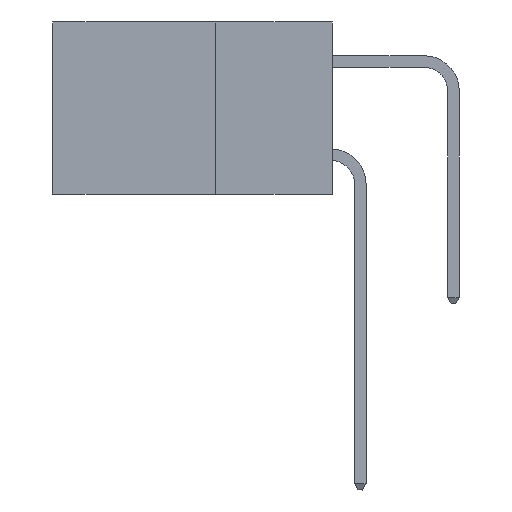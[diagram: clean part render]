
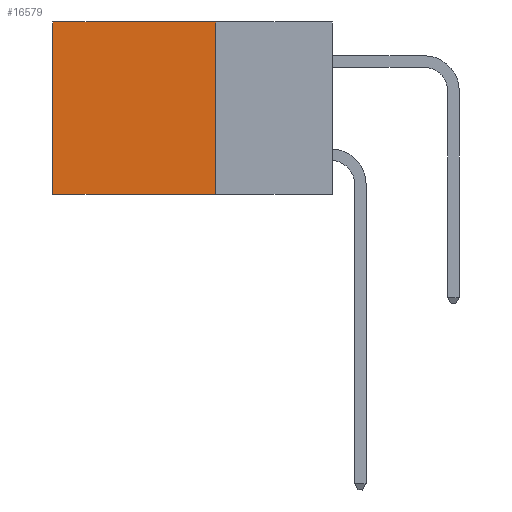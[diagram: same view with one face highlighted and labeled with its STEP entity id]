
A CAD part, left-side view. The second image highlights one B-rep face of the part: STEP entity #16579.
In plain terms, the highlighted planar face has unit normal (-1, 0, 0).
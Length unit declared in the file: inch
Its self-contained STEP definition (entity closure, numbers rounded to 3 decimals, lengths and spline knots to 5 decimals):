
#333 = CARTESIAN_POINT ( 'NONE',  ( 0.298, 0.25, 0. ) ) ;
#1179 = CARTESIAN_POINT ( 'NONE',  ( 0.298, 0.6, 0. ) ) ;
#1319 = VERTEX_POINT ( 'NONE', #1179 ) ;
#2018 = CARTESIAN_POINT ( 'NONE',  ( 0.298, 0.25, 0. ) ) ;
#2697 = VERTEX_POINT ( 'NONE', #4844 ) ;
#3037 = EDGE_LOOP ( 'NONE', ( #7070, #7316, #4612, #20606 ) ) ;
#3149 = LINE ( 'NONE', #3221, #21621 ) ;
#3221 = CARTESIAN_POINT ( 'NONE',  ( 0.298, 0.6, 0. ) ) ;
#4056 = EDGE_CURVE ( 'NONE', #14221, #2697, #16907, .T. ) ;
#4612 = ORIENTED_EDGE ( 'NONE', *, *, #23032, .F. ) ;
#4844 = CARTESIAN_POINT ( 'NONE',  ( 0.298, 0.6, -0.37 ) ) ;
#5186 = EDGE_CURVE ( 'NONE', #1319, #2697, #3149, .T. ) ;
#5882 = FACE_OUTER_BOUND ( 'NONE', #3037, .T. ) ;
#6401 = LINE ( 'NONE', #333, #12344 ) ;
#6707 = EDGE_CURVE ( 'NONE', #17365, #1319, #6401, .T. ) ;
#7070 = ORIENTED_EDGE ( 'NONE', *, *, #5186, .T. ) ;
#7260 = CARTESIAN_POINT ( 'NONE',  ( 0.298, 0.25, 0. ) ) ;
#7316 = ORIENTED_EDGE ( 'NONE', *, *, #4056, .F. ) ;
#7555 = LINE ( 'NONE', #21463, #21176 ) ;
#9073 = DIRECTION ( 'NONE',  ( 1., 0., 0. ) ) ;
#10207 = CARTESIAN_POINT ( 'NONE',  ( 0.298, 0.25, -0.37 ) ) ;
#12268 = VECTOR ( 'NONE', #22583, 39.37008 ) ;
#12344 = VECTOR ( 'NONE', #14803, 39.37008 ) ;
#13038 = CARTESIAN_POINT ( 'NONE',  ( 0.298, 0.25, -0.37 ) ) ;
#14027 = DIRECTION ( 'NONE',  ( 0., 0., -1. ) ) ;
#14221 = VERTEX_POINT ( 'NONE', #13038 ) ;
#14341 = DIRECTION ( 'NONE',  ( 0., 0., -1. ) ) ;
#14803 = DIRECTION ( 'NONE',  ( 0., 1., 0. ) ) ;
#16579 = ADVANCED_FACE ( 'NONE', ( #5882 ), #21402, .F. ) ;
#16907 = LINE ( 'NONE', #10207, #12268 ) ;
#17365 = VERTEX_POINT ( 'NONE', #2018 ) ;
#20606 = ORIENTED_EDGE ( 'NONE', *, *, #6707, .T. ) ;
#20902 = AXIS2_PLACEMENT_3D ( 'NONE', #7260, #9073, #21482 ) ;
#21176 = VECTOR ( 'NONE', #14341, 39.37008 ) ;
#21402 = PLANE ( 'NONE',  #20902 ) ;
#21463 = CARTESIAN_POINT ( 'NONE',  ( 0.298, 0.25, 0. ) ) ;
#21482 = DIRECTION ( 'NONE',  ( 0., 0., -1. ) ) ;
#21621 = VECTOR ( 'NONE', #14027, 39.37008 ) ;
#22583 = DIRECTION ( 'NONE',  ( 0., 1., 0. ) ) ;
#23032 = EDGE_CURVE ( 'NONE', #17365, #14221, #7555, .T. ) ;
